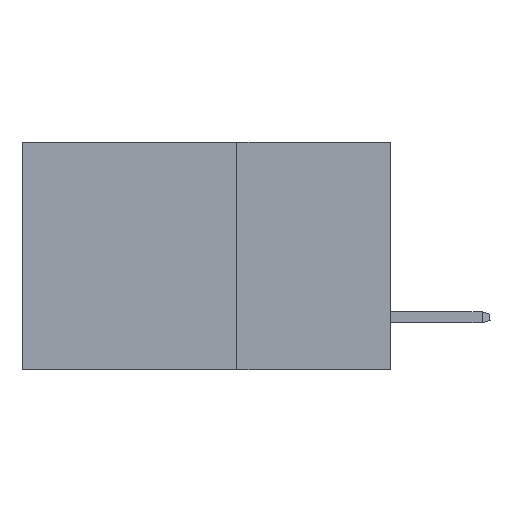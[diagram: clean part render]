
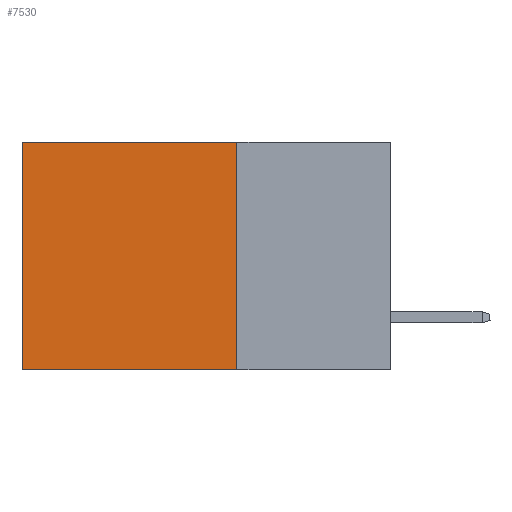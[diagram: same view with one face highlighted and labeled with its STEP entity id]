
A CAD part, left-side view. The second image highlights one B-rep face of the part: STEP entity #7530.
In plain terms, the highlighted planar face has unit normal (-1, 0, 0).
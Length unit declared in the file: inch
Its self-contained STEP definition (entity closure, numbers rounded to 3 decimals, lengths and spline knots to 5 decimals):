
#702 = ORIENTED_EDGE ( 'NONE', *, *, #14946, .T. ) ;
#1632 = PLANE ( 'NONE',  #12246 ) ;
#1694 = VECTOR ( 'NONE', #11738, 39.37008 ) ;
#2005 = VECTOR ( 'NONE', #21328, 39.37008 ) ;
#2152 = DIRECTION ( 'NONE',  ( 0., 1., 0. ) ) ;
#2944 = VERTEX_POINT ( 'NONE', #11962 ) ;
#3563 = VERTEX_POINT ( 'NONE', #22832 ) ;
#3843 = VERTEX_POINT ( 'NONE', #13464 ) ;
#4072 = LINE ( 'NONE', #27737, #2005 ) ;
#5927 = DIRECTION ( 'NONE',  ( 0., 0., -1. ) ) ;
#6542 = EDGE_LOOP ( 'NONE', ( #7090, #9025, #28516, #702 ) ) ;
#7090 = ORIENTED_EDGE ( 'NONE', *, *, #19688, .T. ) ;
#7185 = DIRECTION ( 'NONE',  ( 0., 0., -1. ) ) ;
#7201 = EDGE_CURVE ( 'NONE', #3843, #9312, #13853, .T. ) ;
#7530 = ADVANCED_FACE ( 'NONE', ( #22425 ), #1632, .F. ) ;
#8470 = CARTESIAN_POINT ( 'NONE',  ( 0.2875, 0.25, -0.37 ) ) ;
#9025 = ORIENTED_EDGE ( 'NONE', *, *, #7201, .F. ) ;
#9213 = CARTESIAN_POINT ( 'NONE',  ( 0.2875, 0.6, 0. ) ) ;
#9312 = VERTEX_POINT ( 'NONE', #9722 ) ;
#9722 = CARTESIAN_POINT ( 'NONE',  ( 0.2875, 0.6, -0.37 ) ) ;
#10863 = LINE ( 'NONE', #9213, #17010 ) ;
#11738 = DIRECTION ( 'NONE',  ( 0., 0., -1. ) ) ;
#11962 = CARTESIAN_POINT ( 'NONE',  ( 0.2875, 0.6, 0. ) ) ;
#12246 = AXIS2_PLACEMENT_3D ( 'NONE', #23575, #23670, #5927 ) ;
#13427 = LINE ( 'NONE', #20449, #1694 ) ;
#13464 = CARTESIAN_POINT ( 'NONE',  ( 0.2875, 0.25, -0.37 ) ) ;
#13853 = LINE ( 'NONE', #8470, #21412 ) ;
#14946 = EDGE_CURVE ( 'NONE', #3563, #2944, #4072, .T. ) ;
#17010 = VECTOR ( 'NONE', #7185, 39.37008 ) ;
#17175 = EDGE_CURVE ( 'NONE', #3563, #3843, #13427, .T. ) ;
#19688 = EDGE_CURVE ( 'NONE', #2944, #9312, #10863, .T. ) ;
#20449 = CARTESIAN_POINT ( 'NONE',  ( 0.2875, 0.25, 0. ) ) ;
#21328 = DIRECTION ( 'NONE',  ( 0., 1., 0. ) ) ;
#21412 = VECTOR ( 'NONE', #2152, 39.37008 ) ;
#22425 = FACE_OUTER_BOUND ( 'NONE', #6542, .T. ) ;
#22832 = CARTESIAN_POINT ( 'NONE',  ( 0.2875, 0.25, 0. ) ) ;
#23575 = CARTESIAN_POINT ( 'NONE',  ( 0.2875, 0.25, 0. ) ) ;
#23670 = DIRECTION ( 'NONE',  ( 1., 0., 0. ) ) ;
#27737 = CARTESIAN_POINT ( 'NONE',  ( 0.2875, 0.25, 0. ) ) ;
#28516 = ORIENTED_EDGE ( 'NONE', *, *, #17175, .F. ) ;
